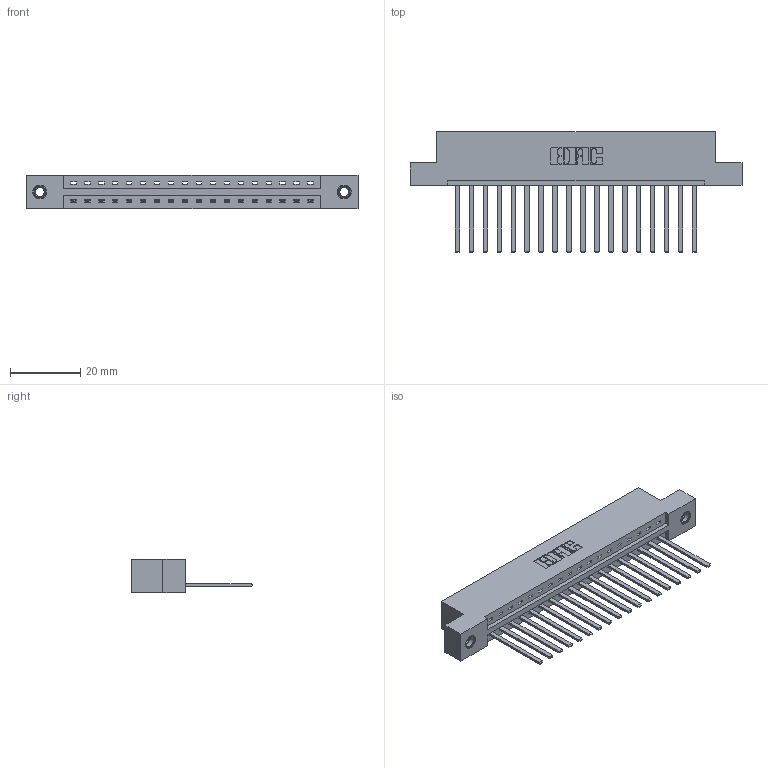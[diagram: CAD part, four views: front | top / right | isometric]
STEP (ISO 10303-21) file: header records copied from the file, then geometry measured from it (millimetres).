
FILE_DESCRIPTION (( 'STEP AP203' ), '1' );
FILE_NAME ('337-018-544-107.STEP', '2018-08-05T01:35:36', ( '' ), ( '' ), 'SwSTEP 2.0', 'SolidWorks 2016', '' );
FILE_SCHEMA (( 'CONFIG_CONTROL_DESIGN' ));
Length unit declared in the file: inch
Products named in the file (4): 345-250-001_345-250-005-103; 337-018-544-107; 337 Part_Flush Mounting Lugs - 0.156 Dia-TI; 345-292-001_345-293-144
Assembly tree (21 placements, depth 2):
  337-018-544-107
    337 Part_Flush Mounting Lugs - 0.156 Dia-TI
    345-292-001_345-293-144  x18
    345-250-001_345-250-005-103  x2
Bounding box: 94.34 x 34.3 x 9.4 mm (x, y, z)
Volume: 9699.2 mm3; surface area: 10616.3 mm2
Topology: 21 solids, 21 shells, 1182 faces, 3507 edges, 2306 vertices
Faces by surface type: plane 858, cylinder 308, cone 12, torus 4
Entity records: 17486 total; most frequent: CARTESIAN_POINT 3023, ORIENTED_EDGE 2970, DIRECTION 2623, EDGE_CURVE 1485, VECTOR 1341, LINE 1341, VERTEX_POINT 984, AXIS2_PLACEMENT_3D 641
